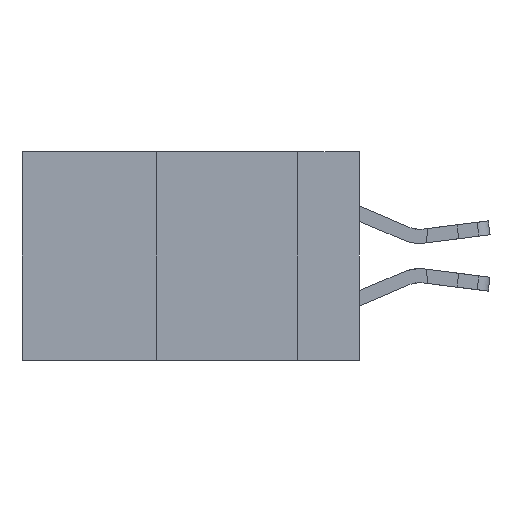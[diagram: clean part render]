
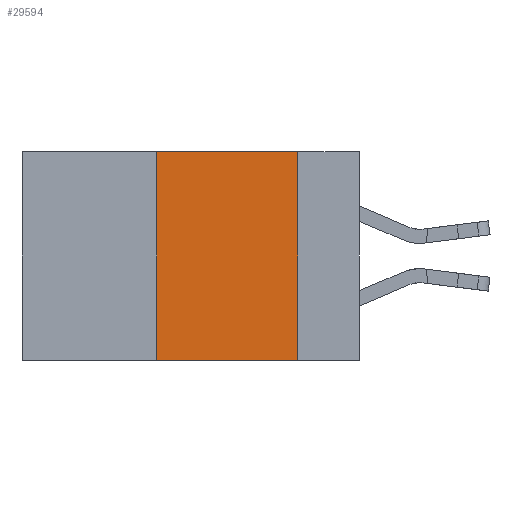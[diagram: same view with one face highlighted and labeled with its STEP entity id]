
A CAD part, left-side view. The second image highlights one B-rep face of the part: STEP entity #29594.
In plain terms, the highlighted planar face has unit normal (-1, 0, 0).
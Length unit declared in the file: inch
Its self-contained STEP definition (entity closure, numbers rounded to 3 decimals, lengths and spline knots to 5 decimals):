
#454 = VERTEX_POINT ( 'NONE', #3939 ) ;
#1349 = VERTEX_POINT ( 'NONE', #22980 ) ;
#1363 = CARTESIAN_POINT ( 'NONE',  ( 0., 0.11, -0.37 ) ) ;
#1517 = EDGE_CURVE ( 'NONE', #31398, #1349, #28458, .T. ) ;
#3665 = EDGE_CURVE ( 'NONE', #454, #19931, #10399, .T. ) ;
#3939 = CARTESIAN_POINT ( 'NONE',  ( 0., 0.36, -0.37 ) ) ;
#5587 = CARTESIAN_POINT ( 'NONE',  ( 0., 0.11, 0. ) ) ;
#7545 = DIRECTION ( 'NONE',  ( 1., 0., 0. ) ) ;
#7787 = VECTOR ( 'NONE', #18620, 39.37008 ) ;
#8178 = DIRECTION ( 'NONE',  ( 0., 0., -1. ) ) ;
#8196 = VECTOR ( 'NONE', #15515, 39.37008 ) ;
#8533 = LINE ( 'NONE', #23752, #7787 ) ;
#10399 = LINE ( 'NONE', #17585, #8196 ) ;
#12884 = CARTESIAN_POINT ( 'NONE',  ( 0., 0.6, 0. ) ) ;
#14260 = EDGE_CURVE ( 'NONE', #1349, #19931, #26825, .T. ) ;
#14933 = ORIENTED_EDGE ( 'NONE', *, *, #14260, .F. ) ;
#15515 = DIRECTION ( 'NONE',  ( 0., -1., 0. ) ) ;
#15877 = CARTESIAN_POINT ( 'NONE',  ( 0., 0.36, 0. ) ) ;
#16887 = EDGE_LOOP ( 'NONE', ( #14933, #22542, #26567, #31866 ) ) ;
#17585 = CARTESIAN_POINT ( 'NONE',  ( 0., 0.6, -0.37 ) ) ;
#17986 = DIRECTION ( 'NONE',  ( 0., 0., -1. ) ) ;
#18620 = DIRECTION ( 'NONE',  ( 0., 0., 1. ) ) ;
#19431 = VECTOR ( 'NONE', #8178, 39.37008 ) ;
#19931 = VERTEX_POINT ( 'NONE', #1363 ) ;
#20536 = PLANE ( 'NONE',  #22534 ) ;
#21152 = VECTOR ( 'NONE', #26554, 39.37008 ) ;
#22534 = AXIS2_PLACEMENT_3D ( 'NONE', #31151, #7545, #17986 ) ;
#22542 = ORIENTED_EDGE ( 'NONE', *, *, #1517, .F. ) ;
#22980 = CARTESIAN_POINT ( 'NONE',  ( 0., 0.11, 0. ) ) ;
#23752 = CARTESIAN_POINT ( 'NONE',  ( 0., 0.36, 0. ) ) ;
#26357 = EDGE_CURVE ( 'NONE', #454, #31398, #8533, .T. ) ;
#26554 = DIRECTION ( 'NONE',  ( 0., -1., 0. ) ) ;
#26567 = ORIENTED_EDGE ( 'NONE', *, *, #26357, .F. ) ;
#26825 = LINE ( 'NONE', #5587, #19431 ) ;
#27900 = FACE_OUTER_BOUND ( 'NONE', #16887, .T. ) ;
#28458 = LINE ( 'NONE', #12884, #21152 ) ;
#29594 = ADVANCED_FACE ( 'NONE', ( #27900 ), #20536, .F. ) ;
#31151 = CARTESIAN_POINT ( 'NONE',  ( 0., 0.6, 0. ) ) ;
#31398 = VERTEX_POINT ( 'NONE', #15877 ) ;
#31866 = ORIENTED_EDGE ( 'NONE', *, *, #3665, .T. ) ;
